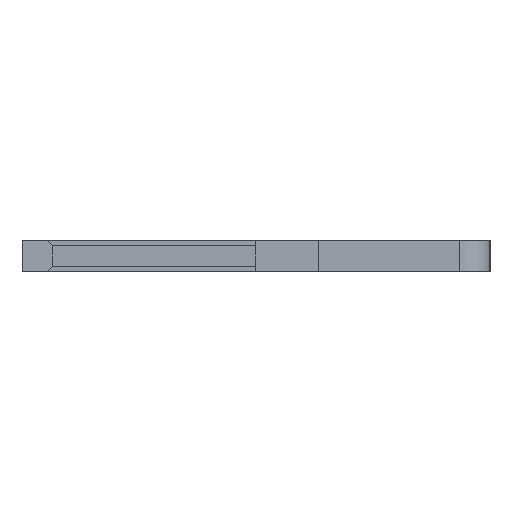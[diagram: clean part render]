
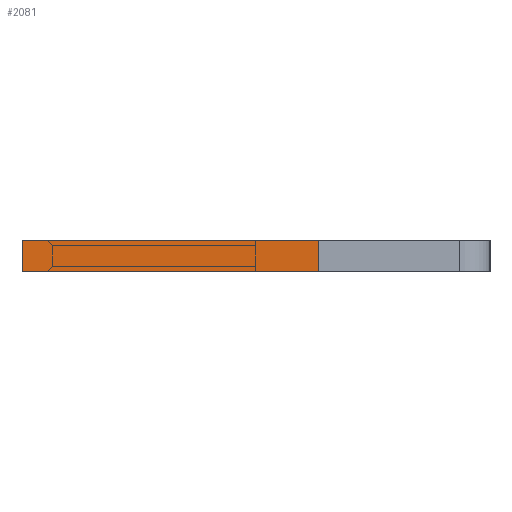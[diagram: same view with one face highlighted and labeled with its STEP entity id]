
A CAD part, left-side view. The second image highlights one B-rep face of the part: STEP entity #2081.
In plain terms, the highlighted face is planar.
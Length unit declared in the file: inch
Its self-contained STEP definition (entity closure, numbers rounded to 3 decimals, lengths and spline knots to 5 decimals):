
#8 = VERTEX_POINT ( 'NONE', #1309 ) ;
#111 = CARTESIAN_POINT ( 'NONE',  ( -0.01, 0.15, -0.04 ) ) ;
#218 = EDGE_LOOP ( 'NONE', ( #1823, #3096, #3358, #1918 ) ) ;
#256 = LINE ( 'NONE', #3241, #3130 ) ;
#461 = PLANE ( 'NONE',  #2655 ) ;
#473 = VECTOR ( 'NONE', #3437, 39.37008 ) ;
#717 = DIRECTION ( 'NONE',  ( 0., 0., 1. ) ) ;
#745 = CARTESIAN_POINT ( 'NONE',  ( 0.01, 0.15, -0.04 ) ) ;
#778 = CARTESIAN_POINT ( 'NONE',  ( 0.01, -0.04, -0.04 ) ) ;
#906 = CARTESIAN_POINT ( 'NONE',  ( -0.01, 0.15, -0.04 ) ) ;
#907 = VECTOR ( 'NONE', #1609, 39.37008 ) ;
#971 = CARTESIAN_POINT ( 'NONE',  ( -0.01, -0.04, -0.04 ) ) ;
#1008 = DIRECTION ( 'NONE',  ( 1., 0., 0. ) ) ;
#1035 = VECTOR ( 'NONE', #3457, 39.37008 ) ;
#1142 = EDGE_CURVE ( 'NONE', #2720, #1241, #2044, .T. ) ;
#1241 = VERTEX_POINT ( 'NONE', #111 ) ;
#1309 = CARTESIAN_POINT ( 'NONE',  ( 0.01, -0.04, -0.04 ) ) ;
#1609 = DIRECTION ( 'NONE',  ( -1., 0., 0. ) ) ;
#1776 = CARTESIAN_POINT ( 'NONE',  ( 0.01, 0.15, -0.04 ) ) ;
#1823 = ORIENTED_EDGE ( 'NONE', *, *, #3289, .T. ) ;
#1877 = CARTESIAN_POINT ( 'NONE',  ( 0.01, 0.15, -0.04 ) ) ;
#1892 = EDGE_CURVE ( 'NONE', #8, #2720, #256, .T. ) ;
#1918 = ORIENTED_EDGE ( 'NONE', *, *, #2260, .T. ) ;
#2044 = LINE ( 'NONE', #1776, #473 ) ;
#2081 = ADVANCED_FACE ( 'NONE', ( #3341 ), #461, .F. ) ;
#2235 = VERTEX_POINT ( 'NONE', #971 ) ;
#2260 = EDGE_CURVE ( 'NONE', #8, #2235, #2594, .T. ) ;
#2594 = LINE ( 'NONE', #778, #907 ) ;
#2655 = AXIS2_PLACEMENT_3D ( 'NONE', #745, #717, #1008 ) ;
#2720 = VERTEX_POINT ( 'NONE', #1877 ) ;
#2969 = DIRECTION ( 'NONE',  ( 0., 1., 0. ) ) ;
#3096 = ORIENTED_EDGE ( 'NONE', *, *, #1142, .F. ) ;
#3130 = VECTOR ( 'NONE', #2969, 39.37008 ) ;
#3241 = CARTESIAN_POINT ( 'NONE',  ( 0.01, 0.15, -0.04 ) ) ;
#3289 = EDGE_CURVE ( 'NONE', #2235, #1241, #3357, .T. ) ;
#3341 = FACE_OUTER_BOUND ( 'NONE', #218, .T. ) ;
#3357 = LINE ( 'NONE', #906, #1035 ) ;
#3358 = ORIENTED_EDGE ( 'NONE', *, *, #1892, .F. ) ;
#3437 = DIRECTION ( 'NONE',  ( -1., 0., 0. ) ) ;
#3457 = DIRECTION ( 'NONE',  ( 0., 1., 0. ) ) ;
